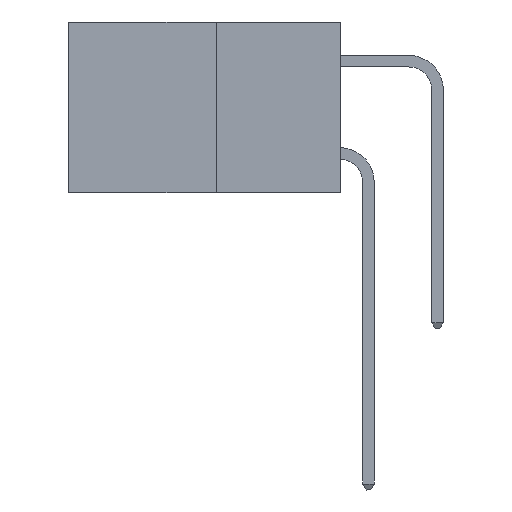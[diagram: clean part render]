
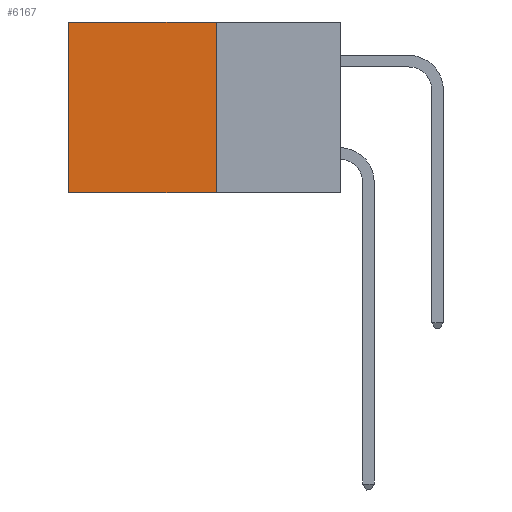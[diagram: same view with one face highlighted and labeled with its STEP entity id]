
A CAD part, left-side view. The second image highlights one B-rep face of the part: STEP entity #6167.
In plain terms, the highlighted planar face has unit normal (-1, 0, 0).
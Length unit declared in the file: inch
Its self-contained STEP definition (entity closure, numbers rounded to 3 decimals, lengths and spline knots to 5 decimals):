
#363 = VECTOR ( 'NONE', #9205, 39.37008 ) ;
#494 = DIRECTION ( 'NONE',  ( 0., 0., -1. ) ) ;
#866 = CARTESIAN_POINT ( 'NONE',  ( 0.277, 0.59, -0.37 ) ) ;
#1011 = PLANE ( 'NONE',  #9107 ) ;
#1097 = VECTOR ( 'NONE', #9438, 39.37008 ) ;
#1124 = EDGE_CURVE ( 'NONE', #7949, #7786, #9525, .T. ) ;
#2442 = EDGE_CURVE ( 'NONE', #3494, #4321, #5074, .T. ) ;
#2546 = DIRECTION ( 'NONE',  ( 0., 0., -1. ) ) ;
#2665 = EDGE_CURVE ( 'NONE', #3494, #7949, #8557, .T. ) ;
#2667 = LINE ( 'NONE', #4937, #363 ) ;
#3494 = VERTEX_POINT ( 'NONE', #9509 ) ;
#4321 = VERTEX_POINT ( 'NONE', #9090 ) ;
#4937 = CARTESIAN_POINT ( 'NONE',  ( 0.277, 0.27, -0.37 ) ) ;
#5074 = LINE ( 'NONE', #6461, #1097 ) ;
#5534 = ORIENTED_EDGE ( 'NONE', *, *, #2442, .F. ) ;
#5636 = ORIENTED_EDGE ( 'NONE', *, *, #7933, .F. ) ;
#6167 = ADVANCED_FACE ( 'NONE', ( #6442 ), #1011, .F. ) ;
#6244 = ORIENTED_EDGE ( 'NONE', *, *, #1124, .T. ) ;
#6256 = CARTESIAN_POINT ( 'NONE',  ( 0.277, 0.27, -0.37 ) ) ;
#6442 = FACE_OUTER_BOUND ( 'NONE', #7978, .T. ) ;
#6443 = CARTESIAN_POINT ( 'NONE',  ( 0.277, 0.59, 0. ) ) ;
#6461 = CARTESIAN_POINT ( 'NONE',  ( 0.277, 0.27, -0.37 ) ) ;
#6504 = ORIENTED_EDGE ( 'NONE', *, *, #2665, .T. ) ;
#6706 = VECTOR ( 'NONE', #8199, 39.37008 ) ;
#6992 = DIRECTION ( 'NONE',  ( 1., 0., 0. ) ) ;
#7708 = VECTOR ( 'NONE', #494, 39.37008 ) ;
#7786 = VERTEX_POINT ( 'NONE', #866 ) ;
#7933 = EDGE_CURVE ( 'NONE', #4321, #7786, #2667, .T. ) ;
#7949 = VERTEX_POINT ( 'NONE', #6443 ) ;
#7978 = EDGE_LOOP ( 'NONE', ( #6244, #5636, #5534, #6504 ) ) ;
#8165 = CARTESIAN_POINT ( 'NONE',  ( 0.277, 0.27, 0. ) ) ;
#8199 = DIRECTION ( 'NONE',  ( 0., 1., 0. ) ) ;
#8557 = LINE ( 'NONE', #8165, #6706 ) ;
#9090 = CARTESIAN_POINT ( 'NONE',  ( 0.277, 0.27, -0.37 ) ) ;
#9107 = AXIS2_PLACEMENT_3D ( 'NONE', #6256, #6992, #2546 ) ;
#9205 = DIRECTION ( 'NONE',  ( 0., 1., 0. ) ) ;
#9438 = DIRECTION ( 'NONE',  ( 0., 0., -1. ) ) ;
#9451 = CARTESIAN_POINT ( 'NONE',  ( 0.277, 0.59, -0.37 ) ) ;
#9509 = CARTESIAN_POINT ( 'NONE',  ( 0.277, 0.27, 0. ) ) ;
#9525 = LINE ( 'NONE', #9451, #7708 ) ;
